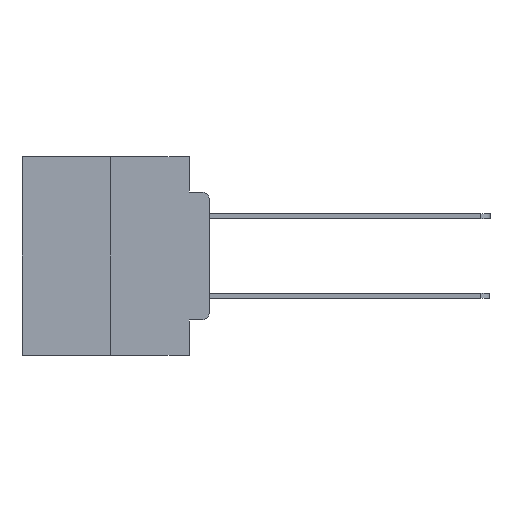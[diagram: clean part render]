
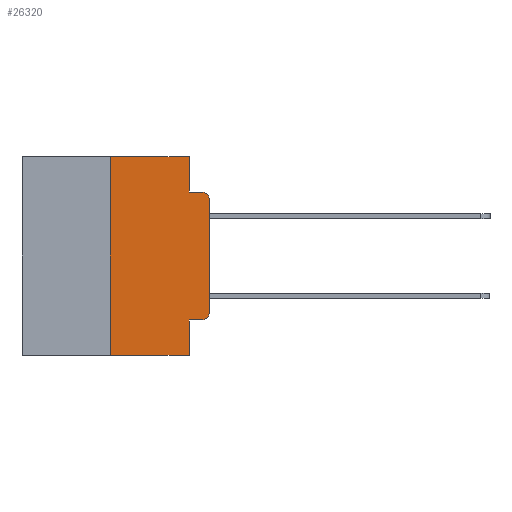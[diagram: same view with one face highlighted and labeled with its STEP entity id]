
A CAD part, left-side view. The second image highlights one B-rep face of the part: STEP entity #26320.
In plain terms, the highlighted planar face has unit normal (-1, 0, 0).
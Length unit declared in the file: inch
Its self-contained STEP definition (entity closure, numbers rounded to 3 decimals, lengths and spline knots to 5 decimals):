
#375 = EDGE_CURVE ( 'NONE', #4647, #18475, #1384, .T. ) ;
#526 = EDGE_CURVE ( 'NONE', #4243, #2339, #26403, .T. ) ;
#723 = VECTOR ( 'NONE', #22536, 39.37008 ) ;
#1014 = ORIENTED_EDGE ( 'NONE', *, *, #8359, .T. ) ;
#1384 = LINE ( 'NONE', #12793, #723 ) ;
#2136 = CARTESIAN_POINT ( 'NONE',  ( 0., 0.051, -0.0885 ) ) ;
#2226 = CARTESIAN_POINT ( 'NONE',  ( 0., 0., -0.3915 ) ) ;
#2339 = VERTEX_POINT ( 'NONE', #6795 ) ;
#3409 = CARTESIAN_POINT ( 'NONE',  ( 0., 0.02, -0.1085 ) ) ;
#3534 = LINE ( 'NONE', #18178, #19895 ) ;
#4243 = VERTEX_POINT ( 'NONE', #9380 ) ;
#4647 = VERTEX_POINT ( 'NONE', #18901 ) ;
#5335 = EDGE_CURVE ( 'NONE', #20497, #24844, #15398, .T. ) ;
#5500 = DIRECTION ( 'NONE',  ( 0., 0., -1. ) ) ;
#5604 = ORIENTED_EDGE ( 'NONE', *, *, #9998, .T. ) ;
#6376 = VECTOR ( 'NONE', #19512, 39.37008 ) ;
#6659 = EDGE_CURVE ( 'NONE', #4243, #17115, #16627, .T. ) ;
#6713 = EDGE_CURVE ( 'NONE', #25373, #18951, #15319, .T. ) ;
#6795 = CARTESIAN_POINT ( 'NONE',  ( 0., 0.051, -0.5 ) ) ;
#6809 = CARTESIAN_POINT ( 'NONE',  ( 0., 0., 0. ) ) ;
#7069 = AXIS2_PLACEMENT_3D ( 'NONE', #3409, #17784, #5500 ) ;
#7297 = CARTESIAN_POINT ( 'NONE',  ( 0., 0.051, -0.4115 ) ) ;
#7495 = CARTESIAN_POINT ( 'NONE',  ( 0., 0.051, 0. ) ) ;
#8021 = VERTEX_POINT ( 'NONE', #7495 ) ;
#8224 = VECTOR ( 'NONE', #22705, 39.37008 ) ;
#8276 = DIRECTION ( 'NONE',  ( 1., 0., 0. ) ) ;
#8359 = EDGE_CURVE ( 'NONE', #17115, #20497, #9898, .T. ) ;
#8559 = CARTESIAN_POINT ( 'NONE',  ( 0., 0.02, -0.3915 ) ) ;
#9081 = CARTESIAN_POINT ( 'NONE',  ( 0., 0.051, 0. ) ) ;
#9380 = CARTESIAN_POINT ( 'NONE',  ( 0., 0.051, -0.4115 ) ) ;
#9591 = DIRECTION ( 'NONE',  ( 0., 0., -1. ) ) ;
#9721 = LINE ( 'NONE', #9081, #25340 ) ;
#9898 = CIRCLE ( 'NONE', #24210, 0.02 ) ;
#9998 = EDGE_CURVE ( 'NONE', #4647, #2339, #25725, .T. ) ;
#10081 = ORIENTED_EDGE ( 'NONE', *, *, #375, .F. ) ;
#10301 = CARTESIAN_POINT ( 'NONE',  ( 0., 0.02, -0.0885 ) ) ;
#10598 = DIRECTION ( 'NONE',  ( 0., 0., -1. ) ) ;
#10926 = DIRECTION ( 'NONE',  ( 0., 0., 1. ) ) ;
#12191 = EDGE_CURVE ( 'NONE', #8021, #25373, #9721, .T. ) ;
#12793 = CARTESIAN_POINT ( 'NONE',  ( 0., 0.25, 0. ) ) ;
#13149 = DIRECTION ( 'NONE',  ( 0., 0., -1. ) ) ;
#14238 = EDGE_CURVE ( 'NONE', #24844, #18951, #18045, .T. ) ;
#14756 = VECTOR ( 'NONE', #10926, 39.37008 ) ;
#14988 = EDGE_CURVE ( 'NONE', #18475, #8021, #3534, .T. ) ;
#15319 = LINE ( 'NONE', #19590, #25516 ) ;
#15398 = LINE ( 'NONE', #6809, #14756 ) ;
#15662 = DIRECTION ( 'NONE',  ( 0., -1., 0. ) ) ;
#16119 = DIRECTION ( 'NONE',  ( 0., -1., 0. ) ) ;
#16293 = AXIS2_PLACEMENT_3D ( 'NONE', #16388, #8276, #22539 ) ;
#16388 = CARTESIAN_POINT ( 'NONE',  ( 0., 0.473, 0. ) ) ;
#16551 = CARTESIAN_POINT ( 'NONE',  ( 0., 0.473, -0.5 ) ) ;
#16627 = LINE ( 'NONE', #7297, #6376 ) ;
#16791 = ORIENTED_EDGE ( 'NONE', *, *, #6713, .F. ) ;
#16929 = CARTESIAN_POINT ( 'NONE',  ( 0., 0.25, 0. ) ) ;
#17115 = VERTEX_POINT ( 'NONE', #22872 ) ;
#17784 = DIRECTION ( 'NONE',  ( -1., 0., 0. ) ) ;
#18045 = CIRCLE ( 'NONE', #7069, 0.02 ) ;
#18178 = CARTESIAN_POINT ( 'NONE',  ( 0., 0.473, 0. ) ) ;
#18475 = VERTEX_POINT ( 'NONE', #16929 ) ;
#18901 = CARTESIAN_POINT ( 'NONE',  ( 0., 0.25, -0.5 ) ) ;
#18951 = VERTEX_POINT ( 'NONE', #10301 ) ;
#19512 = DIRECTION ( 'NONE',  ( 0., -1., 0. ) ) ;
#19590 = CARTESIAN_POINT ( 'NONE',  ( 0., 0.051, -0.0885 ) ) ;
#19642 = ORIENTED_EDGE ( 'NONE', *, *, #14988, .F. ) ;
#19717 = CARTESIAN_POINT ( 'NONE',  ( 0., 0.051, 0. ) ) ;
#19895 = VECTOR ( 'NONE', #16119, 39.37008 ) ;
#19975 = ORIENTED_EDGE ( 'NONE', *, *, #12191, .F. ) ;
#20497 = VERTEX_POINT ( 'NONE', #2226 ) ;
#21778 = FACE_OUTER_BOUND ( 'NONE', #24589, .T. ) ;
#22536 = DIRECTION ( 'NONE',  ( 0., 0., 1. ) ) ;
#22539 = DIRECTION ( 'NONE',  ( 0., 0., -1. ) ) ;
#22705 = DIRECTION ( 'NONE',  ( 0., -1., 0. ) ) ;
#22820 = DIRECTION ( 'NONE',  ( -1., 0., 0. ) ) ;
#22872 = CARTESIAN_POINT ( 'NONE',  ( 0., 0.02, -0.4115 ) ) ;
#23547 = ORIENTED_EDGE ( 'NONE', *, *, #6659, .T. ) ;
#24122 = ORIENTED_EDGE ( 'NONE', *, *, #5335, .T. ) ;
#24210 = AXIS2_PLACEMENT_3D ( 'NONE', #8559, #22820, #10598 ) ;
#24589 = EDGE_LOOP ( 'NONE', ( #24122, #26278, #16791, #19975, #19642, #10081, #5604, #25220, #23547, #1014 ) ) ;
#24844 = VERTEX_POINT ( 'NONE', #25037 ) ;
#25037 = CARTESIAN_POINT ( 'NONE',  ( 0., 0., -0.1085 ) ) ;
#25220 = ORIENTED_EDGE ( 'NONE', *, *, #526, .F. ) ;
#25340 = VECTOR ( 'NONE', #13149, 39.37008 ) ;
#25373 = VERTEX_POINT ( 'NONE', #2136 ) ;
#25516 = VECTOR ( 'NONE', #15662, 39.37008 ) ;
#25725 = LINE ( 'NONE', #16551, #8224 ) ;
#25795 = VECTOR ( 'NONE', #9591, 39.37008 ) ;
#26278 = ORIENTED_EDGE ( 'NONE', *, *, #14238, .T. ) ;
#26320 = ADVANCED_FACE ( 'NONE', ( #21778 ), #26472, .F. ) ;
#26403 = LINE ( 'NONE', #19717, #25795 ) ;
#26472 = PLANE ( 'NONE',  #16293 ) ;
